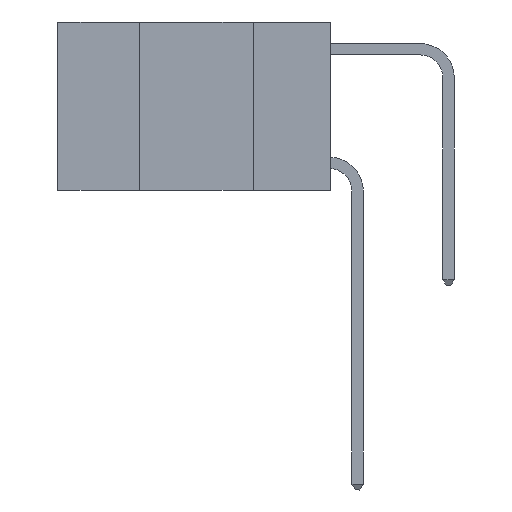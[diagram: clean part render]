
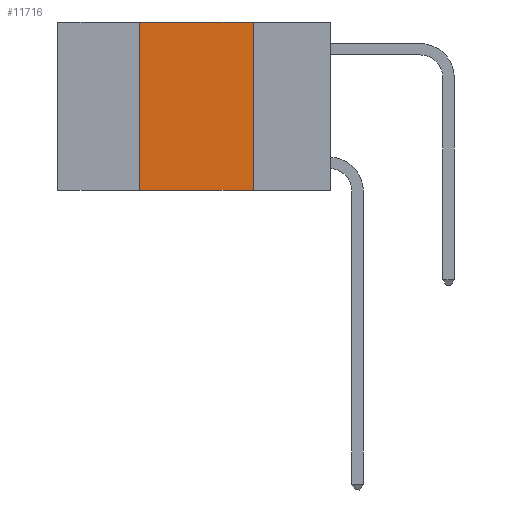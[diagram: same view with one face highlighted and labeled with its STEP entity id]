
A CAD part, left-side view. The second image highlights one B-rep face of the part: STEP entity #11716.
In plain terms, the highlighted planar face has unit normal (-1, 0, 0).
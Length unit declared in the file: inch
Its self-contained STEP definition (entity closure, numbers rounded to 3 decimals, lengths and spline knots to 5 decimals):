
#16 = DIRECTION ( 'NONE',  ( 0., -1., 0. ) ) ;
#327 = CARTESIAN_POINT ( 'NONE',  ( 0., 0.42, 0. ) ) ;
#383 = LINE ( 'NONE', #12048, #12109 ) ;
#679 = DIRECTION ( 'NONE',  ( 0., 0., -1. ) ) ;
#972 = VERTEX_POINT ( 'NONE', #327 ) ;
#2575 = VERTEX_POINT ( 'NONE', #7667 ) ;
#3391 = EDGE_LOOP ( 'NONE', ( #9407, #10895, #9281, #8500 ) ) ;
#3471 = VECTOR ( 'NONE', #679, 39.37008 ) ;
#3953 = EDGE_CURVE ( 'NONE', #5883, #2575, #12146, .T. ) ;
#3963 = DIRECTION ( 'NONE',  ( 0., 0., 1. ) ) ;
#4038 = EDGE_CURVE ( 'NONE', #6526, #972, #4985, .T. ) ;
#4985 = LINE ( 'NONE', #8214, #12557 ) ;
#5530 = EDGE_CURVE ( 'NONE', #972, #5883, #383, .T. ) ;
#5883 = VERTEX_POINT ( 'NONE', #12101 ) ;
#6372 = AXIS2_PLACEMENT_3D ( 'NONE', #6917, #10220, #7803 ) ;
#6526 = VERTEX_POINT ( 'NONE', #11361 ) ;
#6917 = CARTESIAN_POINT ( 'NONE',  ( 0., 0.6, 0. ) ) ;
#7667 = CARTESIAN_POINT ( 'NONE',  ( 0., 0.17, -0.37 ) ) ;
#7803 = DIRECTION ( 'NONE',  ( 0., 0., -1. ) ) ;
#8096 = VECTOR ( 'NONE', #16, 39.37008 ) ;
#8214 = CARTESIAN_POINT ( 'NONE',  ( 0., 0.42, 0. ) ) ;
#8500 = ORIENTED_EDGE ( 'NONE', *, *, #8552, .T. ) ;
#8552 = EDGE_CURVE ( 'NONE', #6526, #2575, #9635, .T. ) ;
#9281 = ORIENTED_EDGE ( 'NONE', *, *, #4038, .F. ) ;
#9407 = ORIENTED_EDGE ( 'NONE', *, *, #3953, .F. ) ;
#9635 = LINE ( 'NONE', #11675, #8096 ) ;
#9949 = DIRECTION ( 'NONE',  ( 0., -1., 0. ) ) ;
#10220 = DIRECTION ( 'NONE',  ( 1., 0., 0. ) ) ;
#10895 = ORIENTED_EDGE ( 'NONE', *, *, #5530, .F. ) ;
#11246 = CARTESIAN_POINT ( 'NONE',  ( 0., 0.17, 0. ) ) ;
#11287 = PLANE ( 'NONE',  #6372 ) ;
#11361 = CARTESIAN_POINT ( 'NONE',  ( 0., 0.42, -0.37 ) ) ;
#11675 = CARTESIAN_POINT ( 'NONE',  ( 0., 0.6, -0.37 ) ) ;
#11716 = ADVANCED_FACE ( 'NONE', ( #12182 ), #11287, .F. ) ;
#12048 = CARTESIAN_POINT ( 'NONE',  ( 0., 0.6, 0. ) ) ;
#12101 = CARTESIAN_POINT ( 'NONE',  ( 0., 0.17, 0. ) ) ;
#12109 = VECTOR ( 'NONE', #9949, 39.37008 ) ;
#12146 = LINE ( 'NONE', #11246, #3471 ) ;
#12182 = FACE_OUTER_BOUND ( 'NONE', #3391, .T. ) ;
#12557 = VECTOR ( 'NONE', #3963, 39.37008 ) ;
